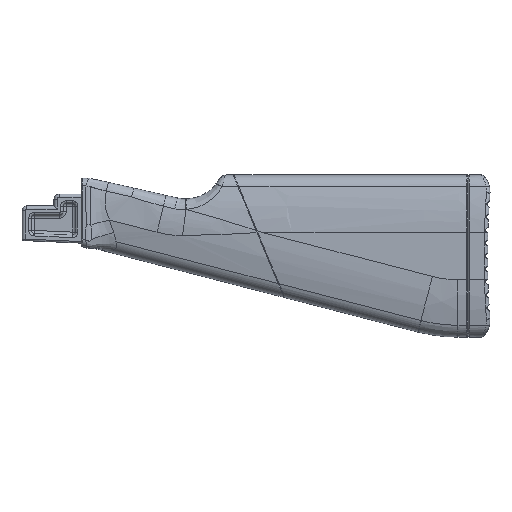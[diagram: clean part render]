
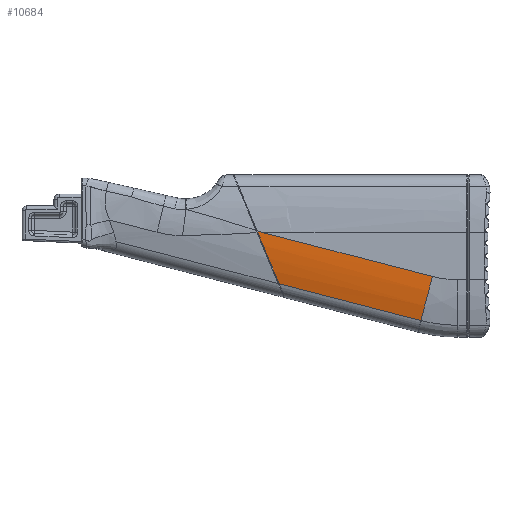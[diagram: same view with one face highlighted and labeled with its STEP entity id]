
A CAD part, left-side view. The second image highlights one B-rep face of the part: STEP entity #10684.
In plain terms, the highlighted cylindrical face has radius 115.186 mm (diameter 230.372 mm), a partial arc.
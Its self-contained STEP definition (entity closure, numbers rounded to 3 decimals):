
#115=ELLIPSE('',#11490,144.239,115.186);
#465=LINE('',#21139,#945);
#488=LINE('',#23078,#968);
#945=VECTOR('',#12740,10.);
#968=VECTOR('',#12909,10.);
#1379=CYLINDRICAL_SURFACE('',#11489,115.186);
#1704=FACE_OUTER_BOUND('',#2424,.T.);
#2424=EDGE_LOOP('',(#7461,#7462,#7463,#7464,#7465));
#3163=CIRCLE('',#11488,115.186);
#3731=B_SPLINE_CURVE_WITH_KNOTS('',3,(#23070,#23071,#23072,#23073,#23074,
#23075),.UNSPECIFIED.,.F.,.F.,(4,2,4),(0.,0.006,
0.231),.UNSPECIFIED.);
#4279=VERTEX_POINT('',#18989);
#4307=VERTEX_POINT('',#21138);
#4378=VERTEX_POINT('',#22964);
#4383=VERTEX_POINT('',#23063);
#4384=VERTEX_POINT('',#23077);
#5405=EDGE_CURVE('',#4307,#4279,#465,.T.);
#5519=EDGE_CURVE('',#4378,#4307,#3163,.T.);
#5521=EDGE_CURVE('',#4279,#4383,#3731,.T.);
#5522=EDGE_CURVE('',#4378,#4384,#488,.T.);
#5523=EDGE_CURVE('',#4383,#4384,#115,.T.);
#7461=ORIENTED_EDGE('',*,*,#5522,.F.);
#7462=ORIENTED_EDGE('',*,*,#5519,.T.);
#7463=ORIENTED_EDGE('',*,*,#5405,.T.);
#7464=ORIENTED_EDGE('',*,*,#5521,.T.);
#7465=ORIENTED_EDGE('',*,*,#5523,.T.);
#10684=ADVANCED_FACE('',(#1704),#1379,.T.);
#11488=AXIS2_PLACEMENT_3D('',#23018,#12905,#12906);
#11489=AXIS2_PLACEMENT_3D('',#23076,#12907,#12908);
#11490=AXIS2_PLACEMENT_3D('',#23079,#12910,#12911);
#12740=DIRECTION('',(0.,0.968,0.25));
#12905=DIRECTION('center_axis',(0.,0.967,0.253));
#12906=DIRECTION('ref_axis',(-0.949,0.08,-0.305));
#12907=DIRECTION('center_axis',(0.,-0.968,-0.25));
#12908=DIRECTION('ref_axis',(-0.949,0.079,-0.305));
#12909=DIRECTION('',(0.,0.968,0.25));
#12910=DIRECTION('center_axis',(0.,-0.924,0.383));
#12911=DIRECTION('ref_axis',(0.,-0.383,-0.924));
#18989=CARTESIAN_POINT('',(84.25,-573.566,96.326));
#21138=CARTESIAN_POINT('',(84.25,-681.487,68.407));
#21139=CARTESIAN_POINT('',(84.25,-681.381,68.434));
#22964=CARTESIAN_POINT('',(87.904,-674.191,40.564));
#23018=CARTESIAN_POINT('Origin',(199.436,-681.487,68.406));
#23063=CARTESIAN_POINT('',(84.253,-571.163,96.152));
#23070=CARTESIAN_POINT('Ctrl Pts',(84.25,-573.566,96.326));
#23071=CARTESIAN_POINT('Ctrl Pts',(84.25,-573.545,96.324));
#23072=CARTESIAN_POINT('Ctrl Pts',(84.25,-573.525,96.323));
#23073=CARTESIAN_POINT('Ctrl Pts',(84.25,-572.723,96.264));
#23074=CARTESIAN_POINT('Ctrl Pts',(84.251,-571.943,96.207));
#23075=CARTESIAN_POINT('Ctrl Pts',(84.253,-571.163,96.152));
#23076=CARTESIAN_POINT('Origin',(199.436,-681.381,68.434));
#23077=CARTESIAN_POINT('',(87.904,-584.587,63.745));
#23078=CARTESIAN_POINT('',(87.904,-530.082,77.846));
#23079=CARTESIAN_POINT('Origin',(199.436,-570.794,97.043));
